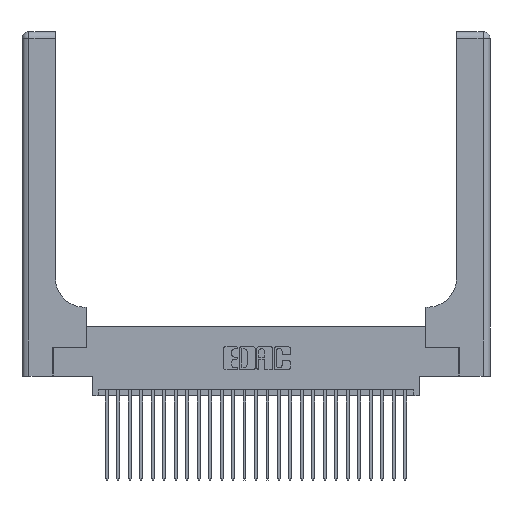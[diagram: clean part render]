
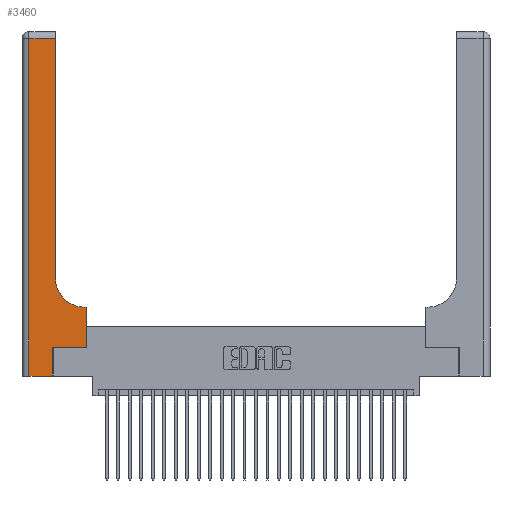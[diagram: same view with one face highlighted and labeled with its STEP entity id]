
A CAD part, top view. The second image highlights one B-rep face of the part: STEP entity #3460.
In plain terms, the highlighted planar face has unit normal (0, 0, 1).
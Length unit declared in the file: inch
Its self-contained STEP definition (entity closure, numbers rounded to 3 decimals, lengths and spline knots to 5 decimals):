
#627 = DIRECTION ( 'NONE',  ( -1., 0., 0. ) ) ;
#872 = EDGE_LOOP ( 'NONE', ( #24010, #10138, #3461, #5938, #2360, #1396, #10812, #19163, #13825 ) ) ;
#888 = AXIS2_PLACEMENT_3D ( 'NONE', #9985, #27385, #14336 ) ;
#1252 = VECTOR ( 'NONE', #8095, 39.37008 ) ;
#1255 = EDGE_CURVE ( 'NONE', #14979, #19035, #8808, .T. ) ;
#1396 = ORIENTED_EDGE ( 'NONE', *, *, #26845, .T. ) ;
#1778 = EDGE_CURVE ( 'NONE', #28108, #9804, #15250, .T. ) ;
#1830 = VECTOR ( 'NONE', #11200, 39.37008 ) ;
#2232 = EDGE_CURVE ( 'NONE', #24528, #6152, #27504, .T. ) ;
#2360 = ORIENTED_EDGE ( 'NONE', *, *, #15528, .T. ) ;
#2997 = CARTESIAN_POINT ( 'NONE',  ( 0.5415, 0.85, 0.37 ) ) ;
#3083 = DIRECTION ( 'NONE',  ( 1., 0., 0. ) ) ;
#3348 = EDGE_CURVE ( 'NONE', #6152, #6391, #7288, .T. ) ;
#3460 = ADVANCED_FACE ( 'NONE', ( #5207 ), #25148, .F. ) ;
#3461 = ORIENTED_EDGE ( 'NONE', *, *, #16611, .T. ) ;
#3625 = CARTESIAN_POINT ( 'NONE',  ( 0.5585, 0.25, 0.37 ) ) ;
#4752 = VECTOR ( 'NONE', #20478, 39.37008 ) ;
#5207 = FACE_OUTER_BOUND ( 'NONE', #872, .T. ) ;
#5219 = DIRECTION ( 'NONE',  ( 1., 0., 0. ) ) ;
#5444 = LINE ( 'NONE', #11797, #4752 ) ;
#5700 = LINE ( 'NONE', #22907, #22409 ) ;
#5938 = ORIENTED_EDGE ( 'NONE', *, *, #1778, .T. ) ;
#6152 = VERTEX_POINT ( 'NONE', #24048 ) ;
#6391 = VERTEX_POINT ( 'NONE', #17924 ) ;
#6653 = CARTESIAN_POINT ( 'NONE',  ( 0.269, 0., 0.37 ) ) ;
#7288 = CIRCLE ( 'NONE', #13373, 0.25 ) ;
#7894 = CARTESIAN_POINT ( 'NONE',  ( 0.06, 0., 0.37 ) ) ;
#8095 = DIRECTION ( 'NONE',  ( 0., 1., 0. ) ) ;
#8549 = VERTEX_POINT ( 'NONE', #12632 ) ;
#8808 = LINE ( 'NONE', #14643, #19674 ) ;
#8995 = CARTESIAN_POINT ( 'NONE',  ( 0.2915, 3., 0.37 ) ) ;
#9525 = VERTEX_POINT ( 'NONE', #27605 ) ;
#9804 = VERTEX_POINT ( 'NONE', #6653 ) ;
#9985 = CARTESIAN_POINT ( 'NONE',  ( 0., 3., 0.37 ) ) ;
#9990 = CARTESIAN_POINT ( 'NONE',  ( 0.06, 2.94, 0.37 ) ) ;
#10138 = ORIENTED_EDGE ( 'NONE', *, *, #1255, .T. ) ;
#10463 = EDGE_CURVE ( 'NONE', #6391, #14979, #19343, .T. ) ;
#10812 = ORIENTED_EDGE ( 'NONE', *, *, #21733, .T. ) ;
#11200 = DIRECTION ( 'NONE',  ( 0., 1., 0. ) ) ;
#11778 = CARTESIAN_POINT ( 'NONE',  ( 0.2915, 0.6, 0.37 ) ) ;
#11797 = CARTESIAN_POINT ( 'NONE',  ( 0.06, 3., 0.37 ) ) ;
#11888 = CARTESIAN_POINT ( 'NONE',  ( 0., 0., 0.37 ) ) ;
#12175 = CARTESIAN_POINT ( 'NONE',  ( 0.2915, 2.94, 0.37 ) ) ;
#12232 = DIRECTION ( 'NONE',  ( 1., 0., 0. ) ) ;
#12632 = CARTESIAN_POINT ( 'NONE',  ( 0.269, 0.25, 0.37 ) ) ;
#13064 = LINE ( 'NONE', #3625, #1252 ) ;
#13373 = AXIS2_PLACEMENT_3D ( 'NONE', #2997, #18319, #5219 ) ;
#13825 = ORIENTED_EDGE ( 'NONE', *, *, #3348, .T. ) ;
#14336 = DIRECTION ( 'NONE',  ( -1., 0., 0. ) ) ;
#14643 = CARTESIAN_POINT ( 'NONE',  ( 0., 2.94, 0.37 ) ) ;
#14979 = VERTEX_POINT ( 'NONE', #12175 ) ;
#15250 = LINE ( 'NONE', #11888, #26119 ) ;
#15528 = EDGE_CURVE ( 'NONE', #9804, #8549, #28416, .T. ) ;
#15906 = VECTOR ( 'NONE', #627, 39.37008 ) ;
#16149 = VECTOR ( 'NONE', #23378, 39.37008 ) ;
#16611 = EDGE_CURVE ( 'NONE', #19035, #28108, #5444, .T. ) ;
#16830 = DIRECTION ( 'NONE',  ( -1., 0., 0. ) ) ;
#17924 = CARTESIAN_POINT ( 'NONE',  ( 0.2915, 0.85, 0.37 ) ) ;
#18319 = DIRECTION ( 'NONE',  ( 0., 0., -1. ) ) ;
#19035 = VERTEX_POINT ( 'NONE', #9990 ) ;
#19042 = CARTESIAN_POINT ( 'NONE',  ( 0.5585, 0.6, 0.37 ) ) ;
#19163 = ORIENTED_EDGE ( 'NONE', *, *, #2232, .T. ) ;
#19343 = LINE ( 'NONE', #8995, #1830 ) ;
#19674 = VECTOR ( 'NONE', #16830, 39.37008 ) ;
#20478 = DIRECTION ( 'NONE',  ( 0., -1., 0. ) ) ;
#21212 = CARTESIAN_POINT ( 'NONE',  ( 0.269, 0., 0.37 ) ) ;
#21733 = EDGE_CURVE ( 'NONE', #9525, #24528, #13064, .T. ) ;
#22409 = VECTOR ( 'NONE', #12232, 39.37008 ) ;
#22907 = CARTESIAN_POINT ( 'NONE',  ( 0.269, 0.25, 0.37 ) ) ;
#23378 = DIRECTION ( 'NONE',  ( 0., 1., 0. ) ) ;
#24010 = ORIENTED_EDGE ( 'NONE', *, *, #10463, .T. ) ;
#24048 = CARTESIAN_POINT ( 'NONE',  ( 0.5415, 0.6, 0.37 ) ) ;
#24528 = VERTEX_POINT ( 'NONE', #19042 ) ;
#25148 = PLANE ( 'NONE',  #888 ) ;
#26119 = VECTOR ( 'NONE', #3083, 39.37008 ) ;
#26845 = EDGE_CURVE ( 'NONE', #8549, #9525, #5700, .T. ) ;
#27385 = DIRECTION ( 'NONE',  ( 0., 0., -1. ) ) ;
#27504 = LINE ( 'NONE', #11778, #15906 ) ;
#27605 = CARTESIAN_POINT ( 'NONE',  ( 0.5585, 0.25, 0.37 ) ) ;
#28108 = VERTEX_POINT ( 'NONE', #7894 ) ;
#28416 = LINE ( 'NONE', #21212, #16149 ) ;
